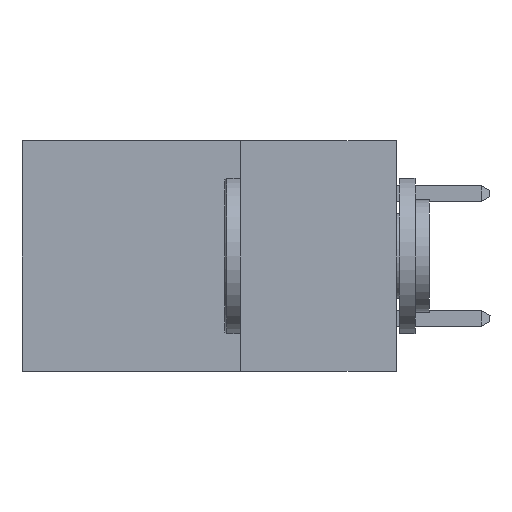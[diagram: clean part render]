
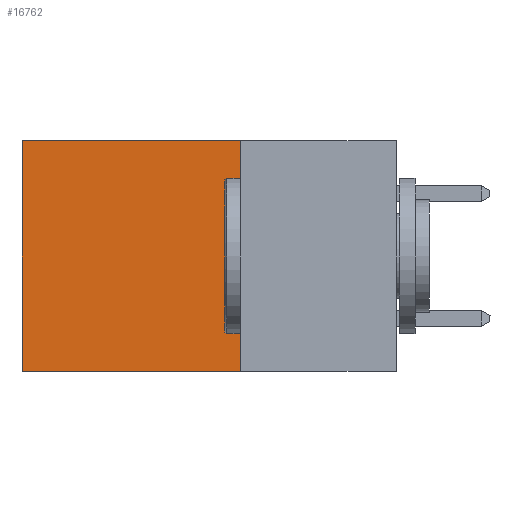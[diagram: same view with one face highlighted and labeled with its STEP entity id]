
A CAD part, left-side view. The second image highlights one B-rep face of the part: STEP entity #16762.
In plain terms, the highlighted planar face has unit normal (-1, 0, 0).
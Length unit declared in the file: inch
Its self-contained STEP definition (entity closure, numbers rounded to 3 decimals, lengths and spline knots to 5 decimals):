
#2617 = CARTESIAN_POINT ( 'NONE',  ( 0.2615, 0.25, -0.37 ) ) ;
#2657 = DIRECTION ( 'NONE',  ( 0., 0., -1. ) ) ;
#4178 = CARTESIAN_POINT ( 'NONE',  ( 0.2615, 0.25, 0. ) ) ;
#4683 = VECTOR ( 'NONE', #18955, 39.37008 ) ;
#5627 = ORIENTED_EDGE ( 'NONE', *, *, #22597, .F. ) ;
#6623 = FACE_OUTER_BOUND ( 'NONE', #26135, .T. ) ;
#7270 = VECTOR ( 'NONE', #8305, 39.37008 ) ;
#8305 = DIRECTION ( 'NONE',  ( 0., 1., 0. ) ) ;
#9422 = EDGE_CURVE ( 'NONE', #16465, #16205, #23274, .T. ) ;
#11973 = CARTESIAN_POINT ( 'NONE',  ( 0.2615, 0.25, 0. ) ) ;
#12455 = ORIENTED_EDGE ( 'NONE', *, *, #21996, .F. ) ;
#12512 = EDGE_CURVE ( 'NONE', #16205, #15626, #19558, .T. ) ;
#13370 = VECTOR ( 'NONE', #14718, 39.37008 ) ;
#13517 = CARTESIAN_POINT ( 'NONE',  ( 0.2615, 0.6, -0.37 ) ) ;
#14296 = CARTESIAN_POINT ( 'NONE',  ( 0.2615, 0.25, -0.37 ) ) ;
#14456 = CARTESIAN_POINT ( 'NONE',  ( 0.2615, 0.25, -0.37 ) ) ;
#14718 = DIRECTION ( 'NONE',  ( 0., 1., 0. ) ) ;
#14851 = DIRECTION ( 'NONE',  ( 1., 0., 0. ) ) ;
#15626 = VERTEX_POINT ( 'NONE', #13517 ) ;
#16205 = VERTEX_POINT ( 'NONE', #17285 ) ;
#16465 = VERTEX_POINT ( 'NONE', #11973 ) ;
#16493 = DIRECTION ( 'NONE',  ( 0., 0., -1. ) ) ;
#16669 = ORIENTED_EDGE ( 'NONE', *, *, #12512, .T. ) ;
#16762 = ADVANCED_FACE ( 'NONE', ( #6623 ), #20820, .F. ) ;
#16966 = CARTESIAN_POINT ( 'NONE',  ( 0.2615, 0.6, -0.37 ) ) ;
#17285 = CARTESIAN_POINT ( 'NONE',  ( 0.2615, 0.6, 0. ) ) ;
#17729 = AXIS2_PLACEMENT_3D ( 'NONE', #18814, #14851, #2657 ) ;
#18814 = CARTESIAN_POINT ( 'NONE',  ( 0.2615, 0.25, -0.37 ) ) ;
#18955 = DIRECTION ( 'NONE',  ( 0., 0., -1. ) ) ;
#19283 = VERTEX_POINT ( 'NONE', #2617 ) ;
#19544 = VECTOR ( 'NONE', #16493, 39.37008 ) ;
#19558 = LINE ( 'NONE', #16966, #4683 ) ;
#20820 = PLANE ( 'NONE',  #17729 ) ;
#21996 = EDGE_CURVE ( 'NONE', #19283, #15626, #25201, .T. ) ;
#22597 = EDGE_CURVE ( 'NONE', #16465, #19283, #25413, .T. ) ;
#23274 = LINE ( 'NONE', #4178, #7270 ) ;
#25201 = LINE ( 'NONE', #14296, #13370 ) ;
#25413 = LINE ( 'NONE', #14456, #19544 ) ;
#25736 = ORIENTED_EDGE ( 'NONE', *, *, #9422, .T. ) ;
#26135 = EDGE_LOOP ( 'NONE', ( #16669, #12455, #5627, #25736 ) ) ;
